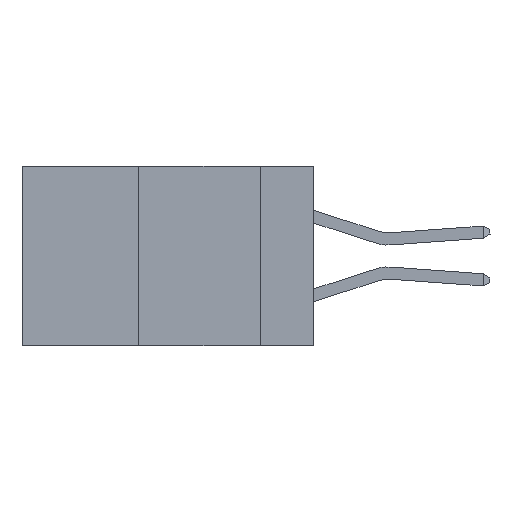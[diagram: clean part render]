
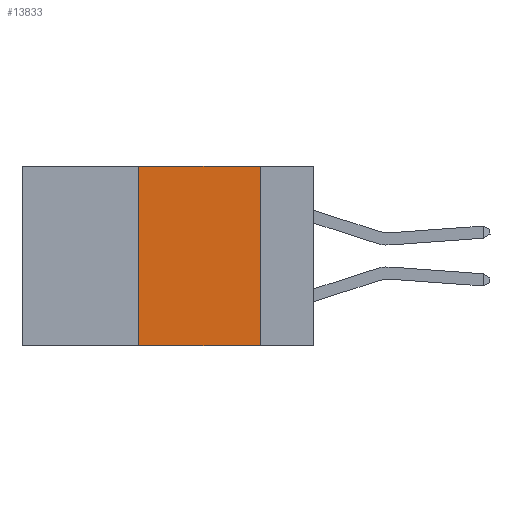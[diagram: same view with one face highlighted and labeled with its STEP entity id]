
A CAD part, left-side view. The second image highlights one B-rep face of the part: STEP entity #13833.
In plain terms, the highlighted planar face has unit normal (-1, 0, 0).
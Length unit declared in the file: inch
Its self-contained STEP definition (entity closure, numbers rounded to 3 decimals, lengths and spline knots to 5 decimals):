
#246 = VERTEX_POINT ( 'NONE', #2549 ) ;
#616 = LINE ( 'NONE', #12718, #5056 ) ;
#1725 = ORIENTED_EDGE ( 'NONE', *, *, #3478, .T. ) ;
#1747 = VECTOR ( 'NONE', #22300, 39.37008 ) ;
#1885 = CARTESIAN_POINT ( 'NONE',  ( 0., 0.36, -0.37 ) ) ;
#2549 = CARTESIAN_POINT ( 'NONE',  ( 0., 0.11, 0. ) ) ;
#3478 = EDGE_CURVE ( 'NONE', #22304, #18114, #616, .T. ) ;
#3790 = FACE_OUTER_BOUND ( 'NONE', #20942, .T. ) ;
#5056 = VECTOR ( 'NONE', #7119, 39.37008 ) ;
#5644 = ORIENTED_EDGE ( 'NONE', *, *, #21003, .F. ) ;
#7119 = DIRECTION ( 'NONE',  ( 0., -1., 0. ) ) ;
#7198 = LINE ( 'NONE', #15774, #7271 ) ;
#7271 = VECTOR ( 'NONE', #17730, 39.37008 ) ;
#7759 = CARTESIAN_POINT ( 'NONE',  ( 0., 0.6, 0. ) ) ;
#8330 = CARTESIAN_POINT ( 'NONE',  ( 0., 0.6, 0. ) ) ;
#8360 = EDGE_CURVE ( 'NONE', #246, #18114, #16132, .T. ) ;
#10656 = DIRECTION ( 'NONE',  ( 0., 0., -1. ) ) ;
#10799 = AXIS2_PLACEMENT_3D ( 'NONE', #7759, #10869, #16457 ) ;
#10869 = DIRECTION ( 'NONE',  ( 1., 0., 0. ) ) ;
#12174 = ORIENTED_EDGE ( 'NONE', *, *, #16032, .F. ) ;
#12718 = CARTESIAN_POINT ( 'NONE',  ( 0., 0.6, -0.37 ) ) ;
#13833 = ADVANCED_FACE ( 'NONE', ( #3790 ), #19564, .F. ) ;
#15088 = LINE ( 'NONE', #8330, #1747 ) ;
#15774 = CARTESIAN_POINT ( 'NONE',  ( 0., 0.36, 0. ) ) ;
#15812 = VERTEX_POINT ( 'NONE', #21176 ) ;
#16032 = EDGE_CURVE ( 'NONE', #15812, #246, #15088, .T. ) ;
#16132 = LINE ( 'NONE', #17865, #22044 ) ;
#16182 = CARTESIAN_POINT ( 'NONE',  ( 0., 0.11, -0.37 ) ) ;
#16457 = DIRECTION ( 'NONE',  ( 0., 0., -1. ) ) ;
#17730 = DIRECTION ( 'NONE',  ( 0., 0., 1. ) ) ;
#17865 = CARTESIAN_POINT ( 'NONE',  ( 0., 0.11, 0. ) ) ;
#18114 = VERTEX_POINT ( 'NONE', #16182 ) ;
#19513 = ORIENTED_EDGE ( 'NONE', *, *, #8360, .F. ) ;
#19564 = PLANE ( 'NONE',  #10799 ) ;
#20942 = EDGE_LOOP ( 'NONE', ( #19513, #12174, #5644, #1725 ) ) ;
#21003 = EDGE_CURVE ( 'NONE', #22304, #15812, #7198, .T. ) ;
#21176 = CARTESIAN_POINT ( 'NONE',  ( 0., 0.36, 0. ) ) ;
#22044 = VECTOR ( 'NONE', #10656, 39.37008 ) ;
#22300 = DIRECTION ( 'NONE',  ( 0., -1., 0. ) ) ;
#22304 = VERTEX_POINT ( 'NONE', #1885 ) ;
